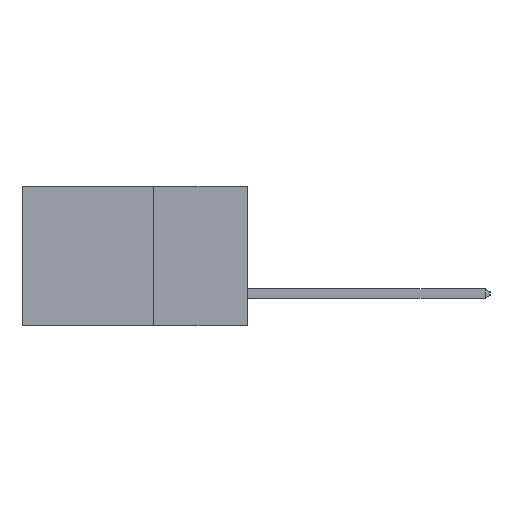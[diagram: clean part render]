
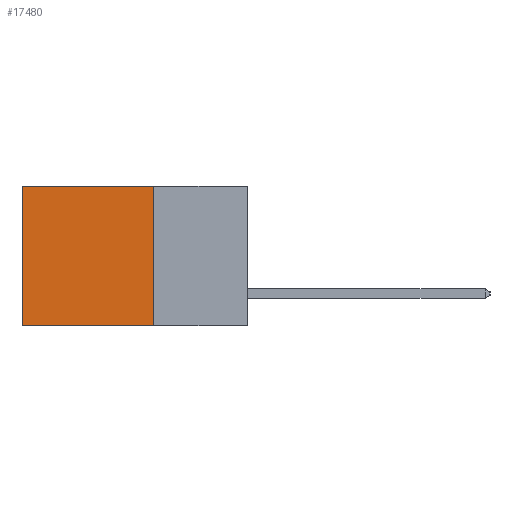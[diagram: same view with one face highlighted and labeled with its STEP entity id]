
A CAD part, left-side view. The second image highlights one B-rep face of the part: STEP entity #17480.
In plain terms, the highlighted planar face has unit normal (-1, 0, 0).
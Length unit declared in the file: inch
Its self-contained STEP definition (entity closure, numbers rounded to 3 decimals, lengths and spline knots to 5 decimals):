
#279 = EDGE_LOOP ( 'NONE', ( #9136, #17260, #1862, #13223 ) ) ;
#817 = EDGE_CURVE ( 'NONE', #11523, #5669, #7528, .T. ) ;
#1058 = EDGE_CURVE ( 'NONE', #7062, #5669, #11288, .T. ) ;
#1862 = ORIENTED_EDGE ( 'NONE', *, *, #9386, .F. ) ;
#2224 = EDGE_CURVE ( 'NONE', #17920, #11523, #3796, .T. ) ;
#2608 = DIRECTION ( 'NONE',  ( 1., 0., 0. ) ) ;
#3343 = VECTOR ( 'NONE', #14617, 39.37008 ) ;
#3796 = LINE ( 'NONE', #12394, #14818 ) ;
#5669 = VERTEX_POINT ( 'NONE', #6749 ) ;
#6749 = CARTESIAN_POINT ( 'NONE',  ( 0.2615, 0.6, -0.37 ) ) ;
#7062 = VERTEX_POINT ( 'NONE', #17164 ) ;
#7528 = LINE ( 'NONE', #13068, #15081 ) ;
#9136 = ORIENTED_EDGE ( 'NONE', *, *, #817, .T. ) ;
#9251 = DIRECTION ( 'NONE',  ( 0., 0., -1. ) ) ;
#9334 = CARTESIAN_POINT ( 'NONE',  ( 0.2615, 0.25, -0.37 ) ) ;
#9386 = EDGE_CURVE ( 'NONE', #17920, #7062, #18038, .T. ) ;
#9675 = AXIS2_PLACEMENT_3D ( 'NONE', #11585, #2608, #13116 ) ;
#10734 = CARTESIAN_POINT ( 'NONE',  ( 0.2615, 0.6, 0. ) ) ;
#11231 = VECTOR ( 'NONE', #9251, 39.37008 ) ;
#11288 = LINE ( 'NONE', #15093, #3343 ) ;
#11523 = VERTEX_POINT ( 'NONE', #10734 ) ;
#11585 = CARTESIAN_POINT ( 'NONE',  ( 0.2615, 0.25, -0.37 ) ) ;
#12394 = CARTESIAN_POINT ( 'NONE',  ( 0.2615, 0.25, 0. ) ) ;
#13068 = CARTESIAN_POINT ( 'NONE',  ( 0.2615, 0.6, -0.37 ) ) ;
#13116 = DIRECTION ( 'NONE',  ( 0., 0., -1. ) ) ;
#13223 = ORIENTED_EDGE ( 'NONE', *, *, #2224, .T. ) ;
#13661 = DIRECTION ( 'NONE',  ( 0., 1., 0. ) ) ;
#13910 = DIRECTION ( 'NONE',  ( 0., 0., -1. ) ) ;
#14211 = CARTESIAN_POINT ( 'NONE',  ( 0.2615, 0.25, 0. ) ) ;
#14617 = DIRECTION ( 'NONE',  ( 0., 1., 0. ) ) ;
#14818 = VECTOR ( 'NONE', #13661, 39.37008 ) ;
#15081 = VECTOR ( 'NONE', #13910, 39.37008 ) ;
#15093 = CARTESIAN_POINT ( 'NONE',  ( 0.2615, 0.25, -0.37 ) ) ;
#16513 = FACE_OUTER_BOUND ( 'NONE', #279, .T. ) ;
#17164 = CARTESIAN_POINT ( 'NONE',  ( 0.2615, 0.25, -0.37 ) ) ;
#17260 = ORIENTED_EDGE ( 'NONE', *, *, #1058, .F. ) ;
#17426 = PLANE ( 'NONE',  #9675 ) ;
#17480 = ADVANCED_FACE ( 'NONE', ( #16513 ), #17426, .F. ) ;
#17920 = VERTEX_POINT ( 'NONE', #14211 ) ;
#18038 = LINE ( 'NONE', #9334, #11231 ) ;
